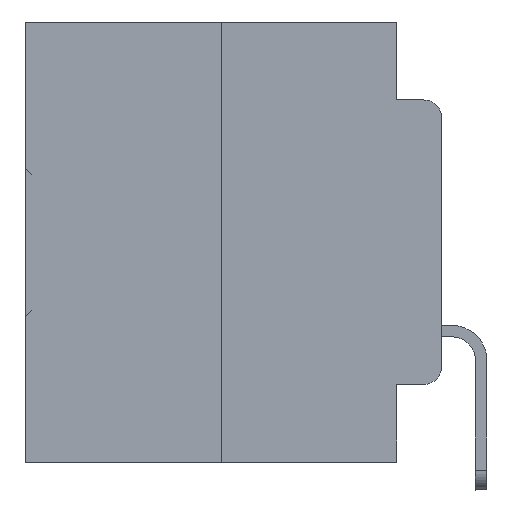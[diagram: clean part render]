
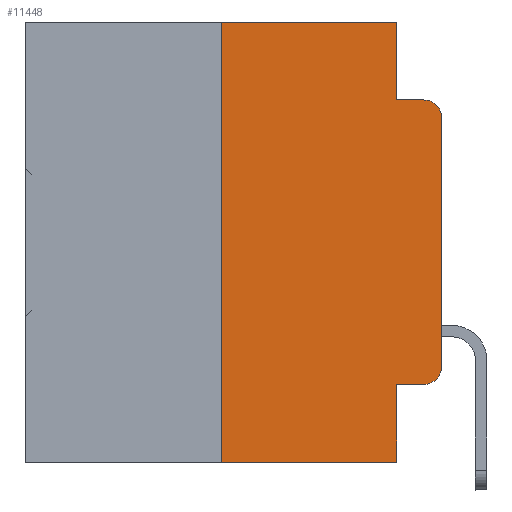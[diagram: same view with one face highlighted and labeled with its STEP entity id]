
A CAD part, left-side view. The second image highlights one B-rep face of the part: STEP entity #11448.
In plain terms, the highlighted planar face has unit normal (-1, 0, 0).
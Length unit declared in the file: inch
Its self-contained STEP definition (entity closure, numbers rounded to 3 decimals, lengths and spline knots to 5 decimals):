
#562 = CIRCLE ( 'NONE', #20274, 0.02 ) ;
#602 = ORIENTED_EDGE ( 'NONE', *, *, #17186, .T. ) ;
#966 = CARTESIAN_POINT ( 'NONE',  ( 0., 0.051, -0.5 ) ) ;
#1043 = EDGE_CURVE ( 'NONE', #27415, #25085, #562, .T. ) ;
#1318 = VERTEX_POINT ( 'NONE', #4219 ) ;
#1573 = VECTOR ( 'NONE', #16091, 39.37008 ) ;
#2356 = LINE ( 'NONE', #13441, #5124 ) ;
#2436 = VERTEX_POINT ( 'NONE', #966 ) ;
#3058 = EDGE_CURVE ( 'NONE', #7746, #21302, #20890, .T. ) ;
#3220 = CARTESIAN_POINT ( 'NONE',  ( 0., 0.051, 0. ) ) ;
#3553 = EDGE_CURVE ( 'NONE', #1318, #2436, #10694, .T. ) ;
#3851 = DIRECTION ( 'NONE',  ( 0., 0., -1. ) ) ;
#4219 = CARTESIAN_POINT ( 'NONE',  ( 0., 0.25, -0.5 ) ) ;
#5000 = LINE ( 'NONE', #29499, #1573 ) ;
#5021 = VECTOR ( 'NONE', #21995, 39.37008 ) ;
#5124 = VECTOR ( 'NONE', #23961, 39.37008 ) ;
#5988 = CARTESIAN_POINT ( 'NONE',  ( 0., 0., -0.3915 ) ) ;
#6859 = DIRECTION ( 'NONE',  ( 0., -1., 0. ) ) ;
#7038 = ORIENTED_EDGE ( 'NONE', *, *, #3058, .T. ) ;
#7746 = VERTEX_POINT ( 'NONE', #18915 ) ;
#7856 = CARTESIAN_POINT ( 'NONE',  ( 0., 0.051, 0. ) ) ;
#8104 = AXIS2_PLACEMENT_3D ( 'NONE', #11479, #19849, #19304 ) ;
#9723 = CARTESIAN_POINT ( 'NONE',  ( 0., 0.25, 0. ) ) ;
#10035 = VERTEX_POINT ( 'NONE', #14281 ) ;
#10143 = VERTEX_POINT ( 'NONE', #9723 ) ;
#10163 = CARTESIAN_POINT ( 'NONE',  ( 0., 0.473, -0.5 ) ) ;
#10615 = DIRECTION ( 'NONE',  ( -1., 0., 0. ) ) ;
#10694 = LINE ( 'NONE', #10163, #12222 ) ;
#11448 = ADVANCED_FACE ( 'NONE', ( #20009 ), #25456, .F. ) ;
#11479 = CARTESIAN_POINT ( 'NONE',  ( 0., 0.473, 0. ) ) ;
#12080 = EDGE_CURVE ( 'NONE', #30834, #25085, #35136, .T. ) ;
#12222 = VECTOR ( 'NONE', #23784, 39.37008 ) ;
#12938 = DIRECTION ( 'NONE',  ( 0., 0., -1. ) ) ;
#13341 = ORIENTED_EDGE ( 'NONE', *, *, #13402, .F. ) ;
#13402 = EDGE_CURVE ( 'NONE', #35577, #2436, #21402, .T. ) ;
#13441 = CARTESIAN_POINT ( 'NONE',  ( 0., 0.25, 0. ) ) ;
#13483 = EDGE_LOOP ( 'NONE', ( #602, #23642, #27058, #13929, #32273, #27634, #24824, #13341, #20059, #7038 ) ) ;
#13929 = ORIENTED_EDGE ( 'NONE', *, *, #19425, .F. ) ;
#14281 = CARTESIAN_POINT ( 'NONE',  ( 0., 0.051, 0. ) ) ;
#15027 = VECTOR ( 'NONE', #12938, 39.37008 ) ;
#15480 = DIRECTION ( 'NONE',  ( -1., 0., 0. ) ) ;
#16091 = DIRECTION ( 'NONE',  ( 0., 0., 1. ) ) ;
#16546 = CARTESIAN_POINT ( 'NONE',  ( 0., 0.473, 0. ) ) ;
#16913 = LINE ( 'NONE', #16546, #5021 ) ;
#17032 = DIRECTION ( 'NONE',  ( 0., 0., -1. ) ) ;
#17186 = EDGE_CURVE ( 'NONE', #21302, #27415, #5000, .T. ) ;
#17389 = CARTESIAN_POINT ( 'NONE',  ( 0., 0., -0.1085 ) ) ;
#18678 = DIRECTION ( 'NONE',  ( 0., -1., 0. ) ) ;
#18856 = VECTOR ( 'NONE', #17032, 39.37008 ) ;
#18915 = CARTESIAN_POINT ( 'NONE',  ( 0., 0.02, -0.4115 ) ) ;
#19167 = CARTESIAN_POINT ( 'NONE',  ( 0., 0.02, -0.1085 ) ) ;
#19304 = DIRECTION ( 'NONE',  ( 0., 0., -1. ) ) ;
#19425 = EDGE_CURVE ( 'NONE', #10035, #30834, #21651, .T. ) ;
#19529 = DIRECTION ( 'NONE',  ( 0., 0., -1. ) ) ;
#19849 = DIRECTION ( 'NONE',  ( 1., 0., 0. ) ) ;
#19906 = EDGE_CURVE ( 'NONE', #1318, #10143, #2356, .T. ) ;
#20009 = FACE_OUTER_BOUND ( 'NONE', #13483, .T. ) ;
#20059 = ORIENTED_EDGE ( 'NONE', *, *, #28529, .T. ) ;
#20274 = AXIS2_PLACEMENT_3D ( 'NONE', #19167, #10615, #19529 ) ;
#20523 = VECTOR ( 'NONE', #18678, 39.37008 ) ;
#20890 = CIRCLE ( 'NONE', #27859, 0.02 ) ;
#21302 = VERTEX_POINT ( 'NONE', #5988 ) ;
#21402 = LINE ( 'NONE', #3220, #18856 ) ;
#21651 = LINE ( 'NONE', #7856, #15027 ) ;
#21995 = DIRECTION ( 'NONE',  ( 0., -1., 0. ) ) ;
#22540 = VECTOR ( 'NONE', #6859, 39.37008 ) ;
#23642 = ORIENTED_EDGE ( 'NONE', *, *, #1043, .T. ) ;
#23784 = DIRECTION ( 'NONE',  ( 0., -1., 0. ) ) ;
#23961 = DIRECTION ( 'NONE',  ( 0., 0., 1. ) ) ;
#24824 = ORIENTED_EDGE ( 'NONE', *, *, #3553, .T. ) ;
#25085 = VERTEX_POINT ( 'NONE', #26348 ) ;
#25456 = PLANE ( 'NONE',  #8104 ) ;
#25922 = LINE ( 'NONE', #26271, #22540 ) ;
#26271 = CARTESIAN_POINT ( 'NONE',  ( 0., 0.051, -0.4115 ) ) ;
#26348 = CARTESIAN_POINT ( 'NONE',  ( 0., 0.02, -0.0885 ) ) ;
#26578 = EDGE_CURVE ( 'NONE', #10143, #10035, #16913, .T. ) ;
#26746 = CARTESIAN_POINT ( 'NONE',  ( 0., 0.051, -0.4115 ) ) ;
#27058 = ORIENTED_EDGE ( 'NONE', *, *, #12080, .F. ) ;
#27415 = VERTEX_POINT ( 'NONE', #17389 ) ;
#27634 = ORIENTED_EDGE ( 'NONE', *, *, #19906, .F. ) ;
#27859 = AXIS2_PLACEMENT_3D ( 'NONE', #29077, #15480, #3851 ) ;
#28529 = EDGE_CURVE ( 'NONE', #35577, #7746, #25922, .T. ) ;
#29077 = CARTESIAN_POINT ( 'NONE',  ( 0., 0.02, -0.3915 ) ) ;
#29499 = CARTESIAN_POINT ( 'NONE',  ( 0., 0., 0. ) ) ;
#30834 = VERTEX_POINT ( 'NONE', #32155 ) ;
#32155 = CARTESIAN_POINT ( 'NONE',  ( 0., 0.051, -0.0885 ) ) ;
#32273 = ORIENTED_EDGE ( 'NONE', *, *, #26578, .F. ) ;
#35136 = LINE ( 'NONE', #35493, #20523 ) ;
#35493 = CARTESIAN_POINT ( 'NONE',  ( 0., 0.051, -0.0885 ) ) ;
#35577 = VERTEX_POINT ( 'NONE', #26746 ) ;
